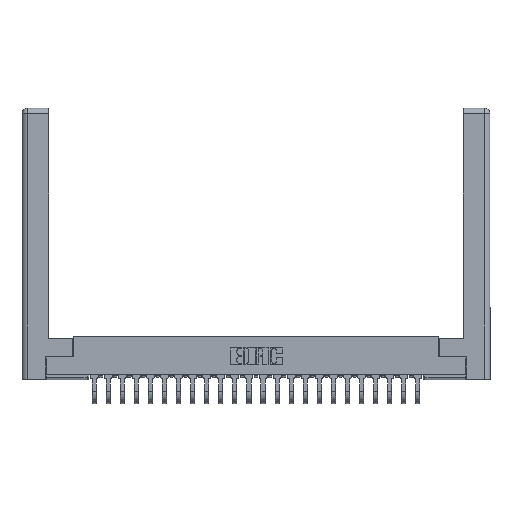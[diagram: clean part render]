
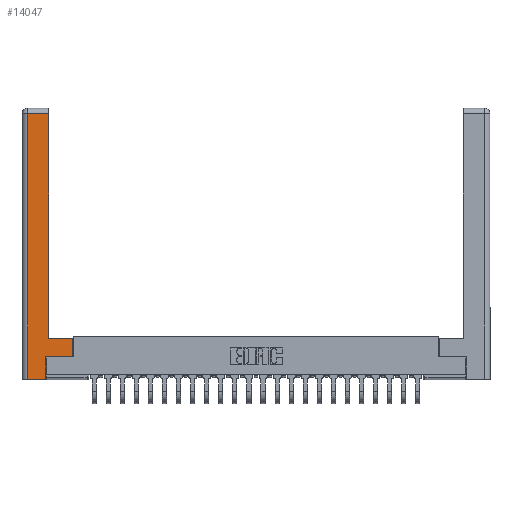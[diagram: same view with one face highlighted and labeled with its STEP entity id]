
A CAD part, top view. The second image highlights one B-rep face of the part: STEP entity #14047.
In plain terms, the highlighted planar face has unit normal (0, 0, 1).
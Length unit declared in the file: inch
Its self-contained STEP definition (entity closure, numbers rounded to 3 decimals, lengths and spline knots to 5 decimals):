
#1167 = CARTESIAN_POINT ( 'NONE',  ( 0.295, 0.45, 0. ) ) ;
#1566 = DIRECTION ( 'NONE',  ( 0., 1., 0. ) ) ;
#1638 = ORIENTED_EDGE ( 'NONE', *, *, #5337, .T. ) ;
#1679 = VECTOR ( 'NONE', #14481, 39.37008 ) ;
#1685 = CARTESIAN_POINT ( 'NONE',  ( 0.265, 0., 0. ) ) ;
#1712 = VECTOR ( 'NONE', #5334, 39.37008 ) ;
#1721 = CARTESIAN_POINT ( 'NONE',  ( 0.265, 0.245, 0. ) ) ;
#2323 = LINE ( 'NONE', #16421, #1679 ) ;
#2329 = DIRECTION ( 'NONE',  ( 0., 0., -1. ) ) ;
#3252 = CARTESIAN_POINT ( 'NONE',  ( 0.565, 0.45, 0. ) ) ;
#3525 = CARTESIAN_POINT ( 'NONE',  ( 0.265, 0., 0. ) ) ;
#3584 = CARTESIAN_POINT ( 'NONE',  ( 0.565, 0.45, 0. ) ) ;
#4396 = CARTESIAN_POINT ( 'NONE',  ( 0.565, 0.245, 0. ) ) ;
#4928 = ORIENTED_EDGE ( 'NONE', *, *, #10409, .T. ) ;
#5317 = LINE ( 'NONE', #15146, #11093 ) ;
#5334 = DIRECTION ( 'NONE',  ( 0., -1., 0. ) ) ;
#5337 = EDGE_CURVE ( 'NONE', #12075, #24808, #19545, .T. ) ;
#5530 = DIRECTION ( 'NONE',  ( 0., 1., 0. ) ) ;
#5565 = DIRECTION ( 'NONE',  ( 0., 1., 0. ) ) ;
#5896 = VECTOR ( 'NONE', #21635, 39.37008 ) ;
#6080 = PLANE ( 'NONE',  #19189 ) ;
#6334 = LINE ( 'NONE', #4396, #7569 ) ;
#7001 = LINE ( 'NONE', #3252, #10661 ) ;
#7051 = ORIENTED_EDGE ( 'NONE', *, *, #12503, .T. ) ;
#7506 = ORIENTED_EDGE ( 'NONE', *, *, #12998, .T. ) ;
#7569 = VECTOR ( 'NONE', #11895, 39.37008 ) ;
#9567 = DIRECTION ( 'NONE',  ( 1., 0., 0. ) ) ;
#9956 = FACE_OUTER_BOUND ( 'NONE', #11567, .T. ) ;
#10409 = EDGE_CURVE ( 'NONE', #24808, #11488, #15649, .T. ) ;
#10541 = EDGE_CURVE ( 'NONE', #18933, #16074, #2323, .T. ) ;
#10661 = VECTOR ( 'NONE', #1566, 39.37008 ) ;
#11093 = VECTOR ( 'NONE', #5565, 39.37008 ) ;
#11237 = CARTESIAN_POINT ( 'NONE',  ( 0.0615, 0., 0. ) ) ;
#11427 = VECTOR ( 'NONE', #5530, 39.37008 ) ;
#11488 = VERTEX_POINT ( 'NONE', #3525 ) ;
#11567 = EDGE_LOOP ( 'NONE', ( #16597, #7051, #1638, #4928, #19936, #7506, #17273, #13691 ) ) ;
#11895 = DIRECTION ( 'NONE',  ( 1., 0., 0. ) ) ;
#11904 = VERTEX_POINT ( 'NONE', #20680 ) ;
#12075 = VERTEX_POINT ( 'NONE', #17307 ) ;
#12503 = EDGE_CURVE ( 'NONE', #13132, #12075, #17627, .T. ) ;
#12998 = EDGE_CURVE ( 'NONE', #23157, #11904, #6334, .T. ) ;
#13132 = VERTEX_POINT ( 'NONE', #22635 ) ;
#13691 = ORIENTED_EDGE ( 'NONE', *, *, #10541, .T. ) ;
#13746 = CARTESIAN_POINT ( 'NONE',  ( 0.0615, 2.94, 0. ) ) ;
#14047 = ADVANCED_FACE ( 'NONE', ( #9956 ), #6080, .F. ) ;
#14481 = DIRECTION ( 'NONE',  ( -1., 0., 0. ) ) ;
#15146 = CARTESIAN_POINT ( 'NONE',  ( 0.265, 0.245, 0. ) ) ;
#15649 = LINE ( 'NONE', #1685, #20679 ) ;
#16074 = VERTEX_POINT ( 'NONE', #1167 ) ;
#16421 = CARTESIAN_POINT ( 'NONE',  ( 0.295, 0.45, 0. ) ) ;
#16597 = ORIENTED_EDGE ( 'NONE', *, *, #23581, .T. ) ;
#17273 = ORIENTED_EDGE ( 'NONE', *, *, #22232, .T. ) ;
#17307 = CARTESIAN_POINT ( 'NONE',  ( 0.0615, 2.94, 0. ) ) ;
#17627 = LINE ( 'NONE', #13746, #5896 ) ;
#17723 = CARTESIAN_POINT ( 'NONE',  ( 0., 0., 0. ) ) ;
#18933 = VERTEX_POINT ( 'NONE', #3584 ) ;
#19177 = CARTESIAN_POINT ( 'NONE',  ( 0.0615, 0., 0. ) ) ;
#19189 = AXIS2_PLACEMENT_3D ( 'NONE', #17723, #2329, #24056 ) ;
#19545 = LINE ( 'NONE', #19177, #1712 ) ;
#19936 = ORIENTED_EDGE ( 'NONE', *, *, #22306, .T. ) ;
#20679 = VECTOR ( 'NONE', #9567, 39.37008 ) ;
#20680 = CARTESIAN_POINT ( 'NONE',  ( 0.565, 0.245, 0. ) ) ;
#21635 = DIRECTION ( 'NONE',  ( -1., 0., 0. ) ) ;
#22232 = EDGE_CURVE ( 'NONE', #11904, #18933, #7001, .T. ) ;
#22306 = EDGE_CURVE ( 'NONE', #11488, #23157, #5317, .T. ) ;
#22635 = CARTESIAN_POINT ( 'NONE',  ( 0.295, 2.94, 0. ) ) ;
#23157 = VERTEX_POINT ( 'NONE', #1721 ) ;
#23369 = LINE ( 'NONE', #25184, #11427 ) ;
#23581 = EDGE_CURVE ( 'NONE', #16074, #13132, #23369, .T. ) ;
#24056 = DIRECTION ( 'NONE',  ( -1., 0., 0. ) ) ;
#24808 = VERTEX_POINT ( 'NONE', #11237 ) ;
#25184 = CARTESIAN_POINT ( 'NONE',  ( 0.295, 3., 0. ) ) ;
